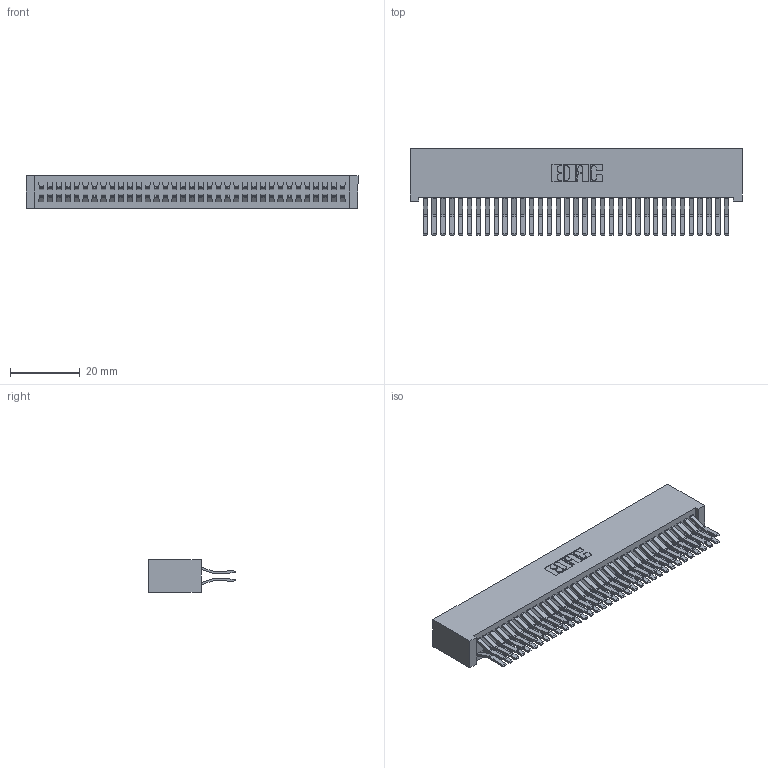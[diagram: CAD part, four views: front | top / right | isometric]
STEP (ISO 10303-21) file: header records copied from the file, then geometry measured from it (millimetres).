
FILE_DESCRIPTION (( 'STEP AP203' ), '1' );
FILE_NAME ('392-070-560-201.STEP', '2019-10-09T12:19:35', ( '' ), ( '' ), 'SwSTEP 2.0', 'SolidWorks 2016', '' );
FILE_SCHEMA (( 'CONFIG_CONTROL_DESIGN' ));
Length unit declared in the file: inch
Products named in the file (3): 342 Part_Lugless; 345-292-001_560 Tail; 392-070-560-201
Assembly tree (71 placements, depth 2):
  392-070-560-201
    342 Part_Lugless
    345-292-001_560 Tail  x70
Bounding box: 95.15 x 24.78 x 9.4 mm (x, y, z)
Volume: 9415 mm3; surface area: 16701 mm2
Topology: 71 solids, 71 shells, 3882 faces, 11545 edges, 7602 vertices
Faces by surface type: plane 2582, cylinder 1300
Entity records: 23101 total; most frequent: CARTESIAN_POINT 3834, ORIENTED_EDGE 3770, DIRECTION 3285, EDGE_CURVE 1885, VECTOR 1761, LINE 1761, VERTEX_POINT 1254, AXIS2_PLACEMENT_3D 762
